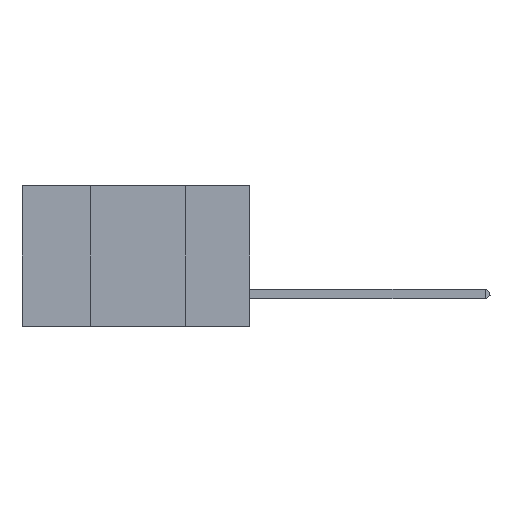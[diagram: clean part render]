
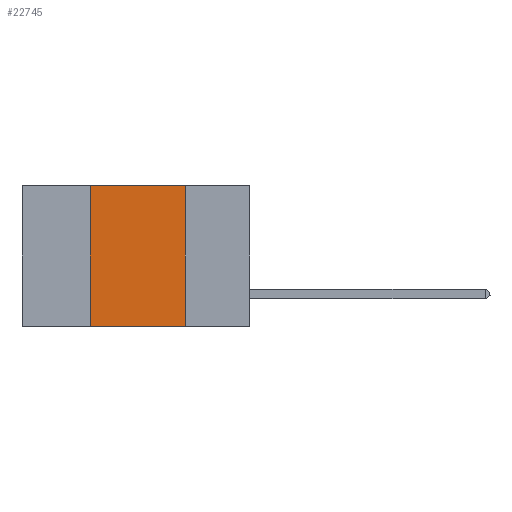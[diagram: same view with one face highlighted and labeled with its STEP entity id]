
A CAD part, left-side view. The second image highlights one B-rep face of the part: STEP entity #22745.
In plain terms, the highlighted planar face has unit normal (-1, 0, 0).
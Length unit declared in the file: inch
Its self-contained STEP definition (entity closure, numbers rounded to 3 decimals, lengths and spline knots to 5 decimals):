
#817 = VERTEX_POINT ( 'NONE', #26749 ) ;
#1519 = DIRECTION ( 'NONE',  ( 0., 0., -1. ) ) ;
#1730 = CARTESIAN_POINT ( 'NONE',  ( 0., 0.42, 0. ) ) ;
#4432 = VECTOR ( 'NONE', #8550, 39.37008 ) ;
#5710 = CARTESIAN_POINT ( 'NONE',  ( 0., 0.6, -0.37 ) ) ;
#8550 = DIRECTION ( 'NONE',  ( 0., -1., 0. ) ) ;
#13450 = DIRECTION ( 'NONE',  ( 0., 0., 1. ) ) ;
#14519 = LINE ( 'NONE', #19882, #4432 ) ;
#16305 = CARTESIAN_POINT ( 'NONE',  ( 0., 0.17, -0.37 ) ) ;
#16776 = ORIENTED_EDGE ( 'NONE', *, *, #41490, .F. ) ;
#18036 = CARTESIAN_POINT ( 'NONE',  ( 0., 0.17, 0. ) ) ;
#18099 = VERTEX_POINT ( 'NONE', #25195 ) ;
#18214 = LINE ( 'NONE', #18036, #19410 ) ;
#18833 = FACE_OUTER_BOUND ( 'NONE', #33199, .T. ) ;
#19410 = VECTOR ( 'NONE', #44556, 39.37008 ) ;
#19882 = CARTESIAN_POINT ( 'NONE',  ( 0., 0.6, 0. ) ) ;
#22251 = VERTEX_POINT ( 'NONE', #16305 ) ;
#22463 = ORIENTED_EDGE ( 'NONE', *, *, #23981, .T. ) ;
#22745 = ADVANCED_FACE ( 'NONE', ( #18833 ), #42668, .F. ) ;
#23905 = CARTESIAN_POINT ( 'NONE',  ( 0., 0.6, 0. ) ) ;
#23981 = EDGE_CURVE ( 'NONE', #817, #22251, #39770, .T. ) ;
#23983 = LINE ( 'NONE', #29066, #44135 ) ;
#25195 = CARTESIAN_POINT ( 'NONE',  ( 0., 0.17, 0. ) ) ;
#26749 = CARTESIAN_POINT ( 'NONE',  ( 0., 0.42, -0.37 ) ) ;
#28522 = VECTOR ( 'NONE', #47679, 39.37008 ) ;
#29066 = CARTESIAN_POINT ( 'NONE',  ( 0., 0.42, 0. ) ) ;
#31568 = DIRECTION ( 'NONE',  ( 1., 0., 0. ) ) ;
#32968 = ORIENTED_EDGE ( 'NONE', *, *, #36041, .F. ) ;
#33183 = EDGE_CURVE ( 'NONE', #817, #36678, #23983, .T. ) ;
#33199 = EDGE_LOOP ( 'NONE', ( #16776, #32968, #35792, #22463 ) ) ;
#35792 = ORIENTED_EDGE ( 'NONE', *, *, #33183, .F. ) ;
#36041 = EDGE_CURVE ( 'NONE', #36678, #18099, #14519, .T. ) ;
#36678 = VERTEX_POINT ( 'NONE', #1730 ) ;
#39770 = LINE ( 'NONE', #5710, #28522 ) ;
#41490 = EDGE_CURVE ( 'NONE', #18099, #22251, #18214, .T. ) ;
#42668 = PLANE ( 'NONE',  #47508 ) ;
#44135 = VECTOR ( 'NONE', #13450, 39.37008 ) ;
#44556 = DIRECTION ( 'NONE',  ( 0., 0., -1. ) ) ;
#47508 = AXIS2_PLACEMENT_3D ( 'NONE', #23905, #31568, #1519 ) ;
#47679 = DIRECTION ( 'NONE',  ( 0., -1., 0. ) ) ;
